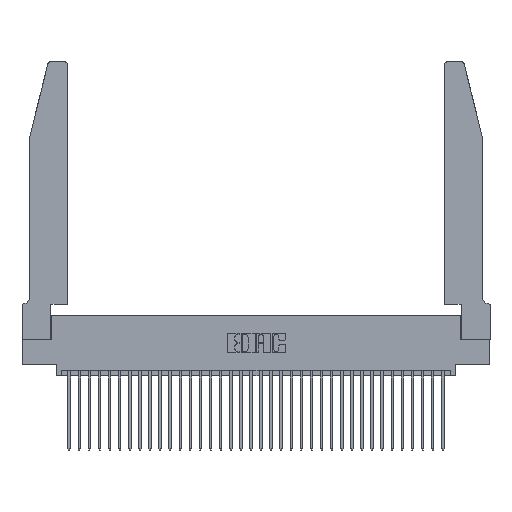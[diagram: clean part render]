
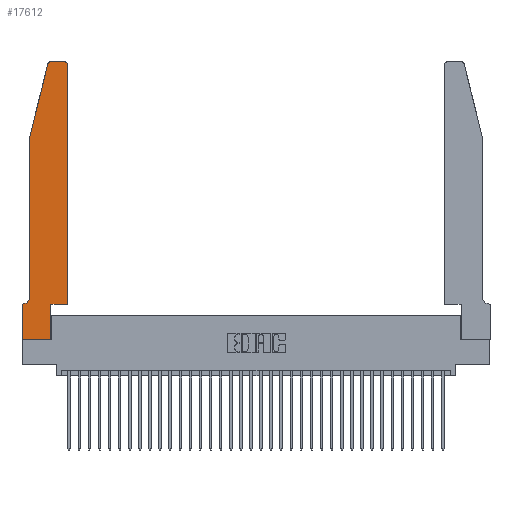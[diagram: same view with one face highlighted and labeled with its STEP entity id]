
A CAD part, top view. The second image highlights one B-rep face of the part: STEP entity #17612.
In plain terms, the highlighted planar face has unit normal (0, 0, 1).
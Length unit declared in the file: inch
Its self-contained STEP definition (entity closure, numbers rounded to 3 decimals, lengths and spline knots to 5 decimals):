
#41 = DIRECTION ( 'NONE',  ( -0.239, -0.971, 0. ) ) ;
#915 = VERTEX_POINT ( 'NONE', #9923 ) ;
#1582 = VERTEX_POINT ( 'NONE', #10449 ) ;
#1758 = EDGE_CURVE ( 'NONE', #33163, #915, #15359, .T. ) ;
#1776 = FACE_OUTER_BOUND ( 'NONE', #12832, .T. ) ;
#3101 = CARTESIAN_POINT ( 'NONE',  ( 0., 0.35, 0.37 ) ) ;
#3103 = DIRECTION ( 'NONE',  ( 0., 1., 0. ) ) ;
#4862 = CARTESIAN_POINT ( 'NONE',  ( 0.0055, 0.35, 0.37 ) ) ;
#4974 = DIRECTION ( 'NONE',  ( 0., 1., 0. ) ) ;
#6105 = CARTESIAN_POINT ( 'NONE',  ( 0.0755, 2., 0.37 ) ) ;
#6167 = DIRECTION ( 'NONE',  ( 0., -1., 0. ) ) ;
#6381 = VECTOR ( 'NONE', #30244, 39.37008 ) ;
#7874 = VECTOR ( 'NONE', #13125, 39.37008 ) ;
#7993 = VERTEX_POINT ( 'NONE', #19079 ) ;
#8567 = PLANE ( 'NONE',  #33458 ) ;
#8679 = CARTESIAN_POINT ( 'NONE',  ( 0.0755, 2., 0.37 ) ) ;
#8686 = DIRECTION ( 'NONE',  ( 1., 0., 0. ) ) ;
#9635 = LINE ( 'NONE', #27980, #30455 ) ;
#9923 = CARTESIAN_POINT ( 'NONE',  ( 0.0755, 2., 0.37 ) ) ;
#10412 = VERTEX_POINT ( 'NONE', #27378 ) ;
#10442 = DIRECTION ( 'NONE',  ( 0., 0., 1. ) ) ;
#10449 = CARTESIAN_POINT ( 'NONE',  ( 0.4205, 2.75, 0.37 ) ) ;
#10569 = CARTESIAN_POINT ( 'NONE',  ( 0.2865, 0., 0.37 ) ) ;
#11359 = VECTOR ( 'NONE', #30301, 39.37008 ) ;
#11478 = EDGE_CURVE ( 'NONE', #1582, #27843, #15228, .T. ) ;
#11531 = ORIENTED_EDGE ( 'NONE', *, *, #26709, .T. ) ;
#11953 = ORIENTED_EDGE ( 'NONE', *, *, #15683, .T. ) ;
#12179 = CARTESIAN_POINT ( 'NONE',  ( 0.0055, 0.42, 0.37 ) ) ;
#12832 = EDGE_LOOP ( 'NONE', ( #31032, #24682, #31868, #11953, #26377, #35189, #15433, #17126, #17981, #11531, #33136, #19662 ) ) ;
#12926 = CIRCLE ( 'NONE', #35276, 0.07 ) ;
#13125 = DIRECTION ( 'NONE',  ( -1., 0., 0. ) ) ;
#13177 = EDGE_CURVE ( 'NONE', #23816, #27557, #28135, .T. ) ;
#14044 = LINE ( 'NONE', #29524, #33046 ) ;
#14158 = CARTESIAN_POINT ( 'NONE',  ( 0.4505, 0.35, 0.37 ) ) ;
#14291 = VERTEX_POINT ( 'NONE', #10569 ) ;
#14964 = DIRECTION ( 'NONE',  ( -1., 0., 0. ) ) ;
#15228 = LINE ( 'NONE', #34702, #7874 ) ;
#15359 = LINE ( 'NONE', #6105, #27146 ) ;
#15433 = ORIENTED_EDGE ( 'NONE', *, *, #30224, .T. ) ;
#15683 = EDGE_CURVE ( 'NONE', #915, #21864, #32616, .T. ) ;
#16538 = CARTESIAN_POINT ( 'NONE',  ( 0.4205, 2.72, 0.37 ) ) ;
#16597 = DIRECTION ( 'NONE',  ( 0., 0., 1. ) ) ;
#16990 = CARTESIAN_POINT ( 'NONE',  ( 0.4505, 0.35, 0.37 ) ) ;
#17126 = ORIENTED_EDGE ( 'NONE', *, *, #30865, .T. ) ;
#17612 = ADVANCED_FACE ( 'NONE', ( #1776 ), #8567, .T. ) ;
#17981 = ORIENTED_EDGE ( 'NONE', *, *, #29248, .T. ) ;
#18612 = CARTESIAN_POINT ( 'NONE',  ( 0.4505, 2.72, 0.37 ) ) ;
#18734 = VERTEX_POINT ( 'NONE', #18612 ) ;
#19079 = CARTESIAN_POINT ( 'NONE',  ( 0.2865, 0.35, 0.37 ) ) ;
#19243 = DIRECTION ( 'NONE',  ( 1., 0., 0. ) ) ;
#19499 = LINE ( 'NONE', #27582, #11359 ) ;
#19662 = ORIENTED_EDGE ( 'NONE', *, *, #26406, .T. ) ;
#20174 = EDGE_CURVE ( 'NONE', #30162, #18734, #24360, .T. ) ;
#20320 = EDGE_CURVE ( 'NONE', #21864, #23816, #12926, .T. ) ;
#20574 = EDGE_CURVE ( 'NONE', #27843, #33163, #27726, .T. ) ;
#21864 = VERTEX_POINT ( 'NONE', #26459 ) ;
#22557 = CARTESIAN_POINT ( 'NONE',  ( 0., 0.35, 0.37 ) ) ;
#23250 = AXIS2_PLACEMENT_3D ( 'NONE', #16538, #16597, #19243 ) ;
#23816 = VERTEX_POINT ( 'NONE', #4862 ) ;
#24360 = LINE ( 'NONE', #16990, #30725 ) ;
#24682 = ORIENTED_EDGE ( 'NONE', *, *, #20574, .T. ) ;
#24987 = DIRECTION ( 'NONE',  ( 0., 0., 1. ) ) ;
#25447 = VECTOR ( 'NONE', #30415, 39.37008 ) ;
#26377 = ORIENTED_EDGE ( 'NONE', *, *, #20320, .T. ) ;
#26406 = EDGE_CURVE ( 'NONE', #18734, #1582, #34076, .T. ) ;
#26459 = CARTESIAN_POINT ( 'NONE',  ( 0.0755, 0.42, 0.37 ) ) ;
#26709 = EDGE_CURVE ( 'NONE', #7993, #30162, #31966, .T. ) ;
#26724 = CARTESIAN_POINT ( 'NONE',  ( 0.284, 2.72, 0.37 ) ) ;
#27146 = VECTOR ( 'NONE', #41, 39.37008 ) ;
#27378 = CARTESIAN_POINT ( 'NONE',  ( 0., 0., 0.37 ) ) ;
#27526 = CARTESIAN_POINT ( 'NONE',  ( 0.0755, 0.35, 0.37 ) ) ;
#27557 = VERTEX_POINT ( 'NONE', #22557 ) ;
#27582 = CARTESIAN_POINT ( 'NONE',  ( 0., 0., 0.37 ) ) ;
#27726 = CIRCLE ( 'NONE', #32849, 0.03 ) ;
#27843 = VERTEX_POINT ( 'NONE', #34290 ) ;
#27980 = CARTESIAN_POINT ( 'NONE',  ( 0., 0., 0.37 ) ) ;
#28135 = LINE ( 'NONE', #27526, #6381 ) ;
#28947 = CARTESIAN_POINT ( 'NONE',  ( 0.25487, 2.72718, 0.37 ) ) ;
#29248 = EDGE_CURVE ( 'NONE', #14291, #7993, #14044, .T. ) ;
#29451 = DIRECTION ( 'NONE',  ( 1., 0., 0. ) ) ;
#29524 = CARTESIAN_POINT ( 'NONE',  ( 0.2865, 0.35, 0.37 ) ) ;
#30162 = VERTEX_POINT ( 'NONE', #14158 ) ;
#30224 = EDGE_CURVE ( 'NONE', #27557, #10412, #9635, .T. ) ;
#30244 = DIRECTION ( 'NONE',  ( -1., 0., 0. ) ) ;
#30301 = DIRECTION ( 'NONE',  ( 1., 0., 0. ) ) ;
#30415 = DIRECTION ( 'NONE',  ( 0., -1., 0. ) ) ;
#30455 = VECTOR ( 'NONE', #6167, 39.37008 ) ;
#30725 = VECTOR ( 'NONE', #3103, 39.37008 ) ;
#30865 = EDGE_CURVE ( 'NONE', #10412, #14291, #19499, .T. ) ;
#31032 = ORIENTED_EDGE ( 'NONE', *, *, #11478, .T. ) ;
#31131 = DIRECTION ( 'NONE',  ( 0., 0., -1. ) ) ;
#31136 = VECTOR ( 'NONE', #34048, 39.37008 ) ;
#31367 = CARTESIAN_POINT ( 'NONE',  ( 0.4505, 0.35, 0.37 ) ) ;
#31868 = ORIENTED_EDGE ( 'NONE', *, *, #1758, .T. ) ;
#31966 = LINE ( 'NONE', #31367, #31136 ) ;
#32616 = LINE ( 'NONE', #8679, #25447 ) ;
#32849 = AXIS2_PLACEMENT_3D ( 'NONE', #26724, #10442, #29451 ) ;
#33046 = VECTOR ( 'NONE', #4974, 39.37008 ) ;
#33136 = ORIENTED_EDGE ( 'NONE', *, *, #20174, .T. ) ;
#33163 = VERTEX_POINT ( 'NONE', #28947 ) ;
#33458 = AXIS2_PLACEMENT_3D ( 'NONE', #3101, #24987, #8686 ) ;
#34048 = DIRECTION ( 'NONE',  ( 1., 0., 0. ) ) ;
#34076 = CIRCLE ( 'NONE', #23250, 0.03 ) ;
#34290 = CARTESIAN_POINT ( 'NONE',  ( 0.284, 2.75, 0.37 ) ) ;
#34702 = CARTESIAN_POINT ( 'NONE',  ( 0.2605, 2.75, 0.37 ) ) ;
#35189 = ORIENTED_EDGE ( 'NONE', *, *, #13177, .T. ) ;
#35276 = AXIS2_PLACEMENT_3D ( 'NONE', #12179, #31131, #14964 ) ;
